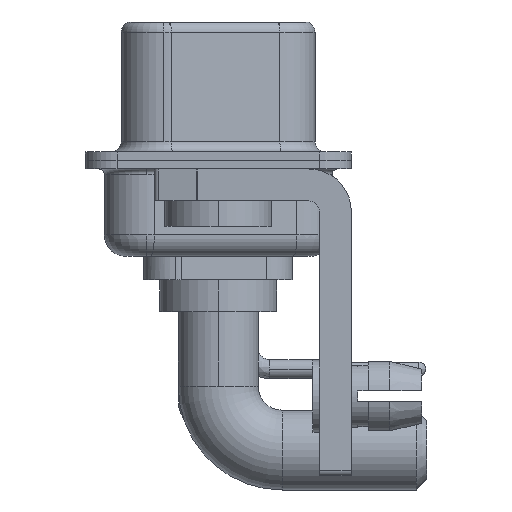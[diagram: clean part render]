
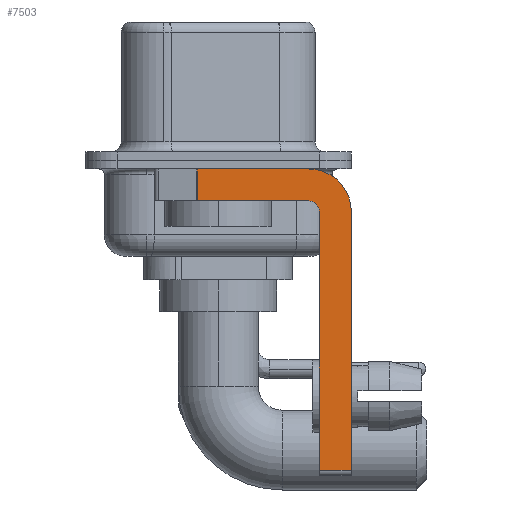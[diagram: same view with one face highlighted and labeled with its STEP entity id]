
A CAD part, left-side view. The second image highlights one B-rep face of the part: STEP entity #7503.
In plain terms, the highlighted planar face has unit normal (-1, 0, 0).
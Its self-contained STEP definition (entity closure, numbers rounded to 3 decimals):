
#301 = ORIENTED_EDGE ( 'NONE', *, *, #2487, .T. ) ;
#369 = ORIENTED_EDGE ( 'NONE', *, *, #8805, .F. ) ;
#702 = AXIS2_PLACEMENT_3D ( 'NONE', #24949, #5408, #14115 ) ;
#1626 = LINE ( 'NONE', #17166, #3341 ) ;
#1686 = EDGE_CURVE ( 'NONE', #5734, #5040, #16353, .T. ) ;
#2475 = VECTOR ( 'NONE', #15022, 1000. ) ;
#2487 = EDGE_CURVE ( 'NONE', #27371, #19167, #1626, .T. ) ;
#2782 = CARTESIAN_POINT ( 'NONE',  ( -2.9, 0.978, -0.4 ) ) ;
#3128 = DIRECTION ( 'NONE',  ( 0., 0., -1. ) ) ;
#3341 = VECTOR ( 'NONE', #6179, 1000. ) ;
#3653 = DIRECTION ( 'NONE',  ( 0., 0., -1. ) ) ;
#4513 = ORIENTED_EDGE ( 'NONE', *, *, #17065, .T. ) ;
#4564 = VECTOR ( 'NONE', #3653, 1000. ) ;
#4692 = LINE ( 'NONE', #22091, #26275 ) ;
#4710 = ORIENTED_EDGE ( 'NONE', *, *, #6654, .F. ) ;
#4828 = DIRECTION ( 'NONE',  ( 0., 1., 0. ) ) ;
#4938 = CARTESIAN_POINT ( 'NONE',  ( -2.9, -4.25, -1.9 ) ) ;
#5040 = VERTEX_POINT ( 'NONE', #14713 ) ;
#5408 = DIRECTION ( 'NONE',  ( 1., 0., 0. ) ) ;
#5677 = CARTESIAN_POINT ( 'NONE',  ( -2.9, 0.978, -1.9 ) ) ;
#5734 = VERTEX_POINT ( 'NONE', #10553 ) ;
#6001 = CARTESIAN_POINT ( 'NONE',  ( -2.9, -4.75, -14.55 ) ) ;
#6179 = DIRECTION ( 'NONE',  ( 0., 0., -1. ) ) ;
#6654 = EDGE_CURVE ( 'NONE', #27371, #9138, #14461, .T. ) ;
#7451 = ORIENTED_EDGE ( 'NONE', *, *, #27442, .F. ) ;
#7503 = ADVANCED_FACE ( 'NONE', ( #20526 ), #7547, .F. ) ;
#7547 = PLANE ( 'NONE',  #702 ) ;
#8805 = EDGE_CURVE ( 'NONE', #9138, #5734, #26277, .T. ) ;
#9138 = VERTEX_POINT ( 'NONE', #26060 ) ;
#9179 = VERTEX_POINT ( 'NONE', #4938 ) ;
#9797 = CARTESIAN_POINT ( 'NONE',  ( -2.9, -4.25, -2.4 ) ) ;
#10553 = CARTESIAN_POINT ( 'NONE',  ( -2.9, -6.25, -2.4 ) ) ;
#10739 = EDGE_CURVE ( 'NONE', #9179, #19167, #4692, .T. ) ;
#12710 = DIRECTION ( 'NONE',  ( 0., -1., 0. ) ) ;
#13502 = VERTEX_POINT ( 'NONE', #14686 ) ;
#13998 = AXIS2_PLACEMENT_3D ( 'NONE', #26949, #27087, #3128 ) ;
#14115 = DIRECTION ( 'NONE',  ( 0., 0., -1. ) ) ;
#14221 = CARTESIAN_POINT ( 'NONE',  ( -2.9, -6.25, -2.4 ) ) ;
#14461 = LINE ( 'NONE', #14606, #2475 ) ;
#14569 = CARTESIAN_POINT ( 'NONE',  ( -2.9, -4.25, -14.55 ) ) ;
#14606 = CARTESIAN_POINT ( 'NONE',  ( -2.9, 3., -0.4 ) ) ;
#14686 = CARTESIAN_POINT ( 'NONE',  ( -2.9, -4.75, -2.4 ) ) ;
#14713 = CARTESIAN_POINT ( 'NONE',  ( -2.9, -6.25, -14.55 ) ) ;
#15022 = DIRECTION ( 'NONE',  ( 0., -1., 0. ) ) ;
#15039 = ORIENTED_EDGE ( 'NONE', *, *, #1686, .F. ) ;
#15354 = ORIENTED_EDGE ( 'NONE', *, *, #17883, .F. ) ;
#15783 = EDGE_LOOP ( 'NONE', ( #4710, #301, #18646, #7451, #15354, #4513, #15039, #369 ) ) ;
#16353 = LINE ( 'NONE', #14221, #4564 ) ;
#16757 = DIRECTION ( 'NONE',  ( 0., 0., 1. ) ) ;
#17026 = VERTEX_POINT ( 'NONE', #6001 ) ;
#17065 = EDGE_CURVE ( 'NONE', #17026, #5040, #23108, .T. ) ;
#17166 = CARTESIAN_POINT ( 'NONE',  ( -2.9, 0.978, -1.9 ) ) ;
#17883 = EDGE_CURVE ( 'NONE', #17026, #13502, #18226, .T. ) ;
#18226 = LINE ( 'NONE', #21179, #23553 ) ;
#18646 = ORIENTED_EDGE ( 'NONE', *, *, #10739, .F. ) ;
#19167 = VERTEX_POINT ( 'NONE', #5677 ) ;
#20526 = FACE_OUTER_BOUND ( 'NONE', #15783, .T. ) ;
#21176 = AXIS2_PLACEMENT_3D ( 'NONE', #9797, #27184, #24759 ) ;
#21179 = CARTESIAN_POINT ( 'NONE',  ( -2.9, -4.75, -14.8 ) ) ;
#22091 = CARTESIAN_POINT ( 'NONE',  ( -2.9, -4.25, -1.9 ) ) ;
#23108 = LINE ( 'NONE', #14569, #23858 ) ;
#23459 = CIRCLE ( 'NONE', #21176, 0.5 ) ;
#23553 = VECTOR ( 'NONE', #16757, 1000. ) ;
#23858 = VECTOR ( 'NONE', #12710, 1000. ) ;
#24759 = DIRECTION ( 'NONE',  ( 0., 0., 1. ) ) ;
#24949 = CARTESIAN_POINT ( 'NONE',  ( -2.9, -4.25, -2.4 ) ) ;
#26060 = CARTESIAN_POINT ( 'NONE',  ( -2.9, -4.25, -0.4 ) ) ;
#26275 = VECTOR ( 'NONE', #4828, 1000. ) ;
#26277 = CIRCLE ( 'NONE', #13998, 2. ) ;
#26949 = CARTESIAN_POINT ( 'NONE',  ( -2.9, -4.25, -2.4 ) ) ;
#27087 = DIRECTION ( 'NONE',  ( 1., 0., 0. ) ) ;
#27184 = DIRECTION ( 'NONE',  ( -1., 0., 0. ) ) ;
#27371 = VERTEX_POINT ( 'NONE', #2782 ) ;
#27442 = EDGE_CURVE ( 'NONE', #13502, #9179, #23459, .T. ) ;
